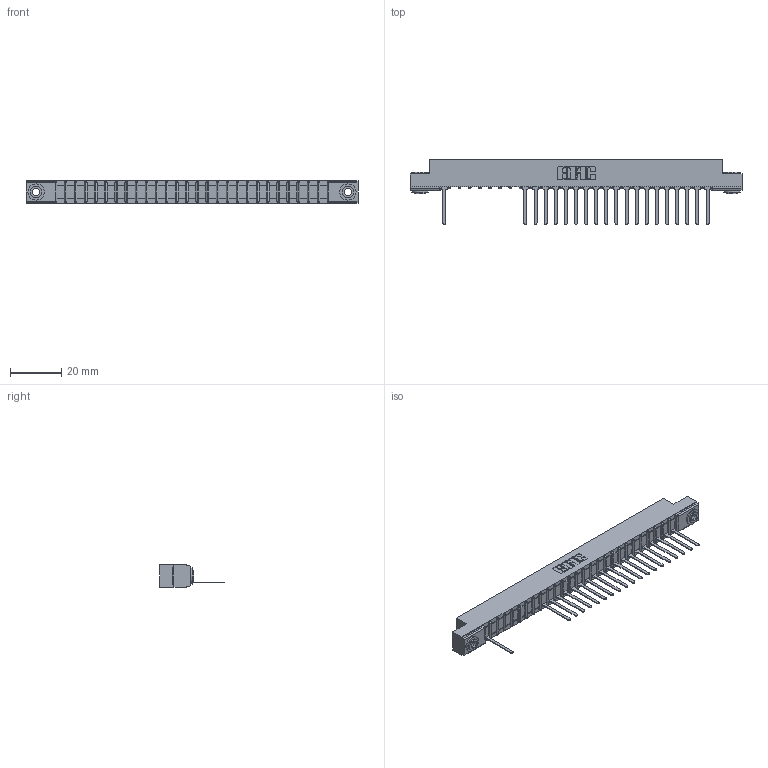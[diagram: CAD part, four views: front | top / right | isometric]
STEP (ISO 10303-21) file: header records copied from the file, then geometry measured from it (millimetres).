
FILE_DESCRIPTION (( 'STEP AP203' ), '1' );
FILE_NAME ('307-027-547-103.STEP', '2018-08-04T15:08:58', ( '' ), ( '' ), 'SwSTEP 2.0', 'SolidWorks 2016', '' );
FILE_SCHEMA (( 'CONFIG_CONTROL_DESIGN' ));
Length unit declared in the file: inch
Products named in the file (4): 307-290-001_547; 345-250-002_345-250-002-102; 307-027-547-103; 307 Part_.156 Dia Mounting Holes
Assembly tree (23 placements, depth 2):
  307-027-547-103
    307 Part_.156 Dia Mounting Holes
    307-290-001_547  x20
    345-250-002_345-250-002-102  x2
Bounding box: 130 x 25.43 x 8.71 mm (x, y, z)
Volume: 8141 mm3; surface area: 12718.9 mm2
Topology: 23 solids, 23 shells, 1458 faces, 4123 edges, 2642 vertices
Faces by surface type: plane 918, cylinder 476, sphere 56, cone 8
Entity records: 25805 total; most frequent: CARTESIAN_POINT 4350, ORIENTED_EDGE 4334, DIRECTION 4247, EDGE_CURVE 2167, LINE 1649, VECTOR 1649, VERTEX_POINT 1402, AXIS2_PLACEMENT_3D 1299
